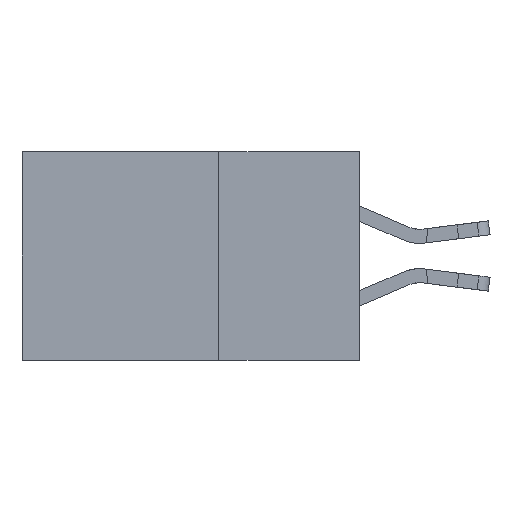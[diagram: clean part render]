
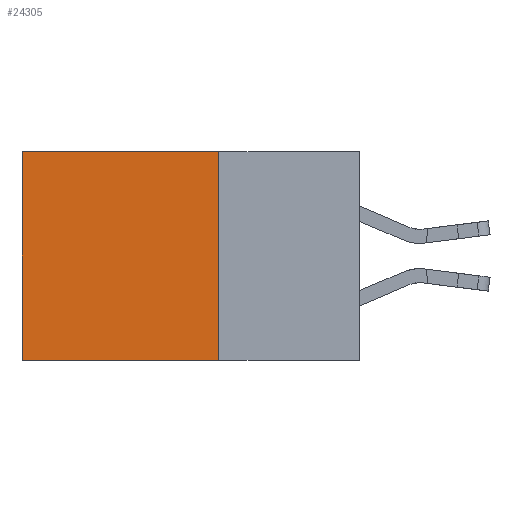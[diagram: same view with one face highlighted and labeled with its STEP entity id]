
A CAD part, left-side view. The second image highlights one B-rep face of the part: STEP entity #24305.
In plain terms, the highlighted planar face has unit normal (-1, 0, 0).
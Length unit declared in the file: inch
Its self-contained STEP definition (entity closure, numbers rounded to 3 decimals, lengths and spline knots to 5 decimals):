
#8 = DIRECTION ( 'NONE',  ( 0., 0., -1. ) ) ;
#394 = EDGE_CURVE ( 'NONE', #16042, #1159, #5912, .T. ) ;
#1159 = VERTEX_POINT ( 'NONE', #7861 ) ;
#1771 = AXIS2_PLACEMENT_3D ( 'NONE', #2518, #14884, #28732 ) ;
#2518 = CARTESIAN_POINT ( 'NONE',  ( 0.2875, 0.25, 0. ) ) ;
#3125 = VECTOR ( 'NONE', #8450, 39.37008 ) ;
#4966 = ORIENTED_EDGE ( 'NONE', *, *, #394, .F. ) ;
#4973 = EDGE_CURVE ( 'NONE', #1159, #19382, #18060, .T. ) ;
#5912 = LINE ( 'NONE', #15812, #14977 ) ;
#7436 = FACE_OUTER_BOUND ( 'NONE', #29350, .T. ) ;
#7861 = CARTESIAN_POINT ( 'NONE',  ( 0.2875, 0.25, -0.37 ) ) ;
#8338 = CARTESIAN_POINT ( 'NONE',  ( 0.2875, 0.25, 0. ) ) ;
#8450 = DIRECTION ( 'NONE',  ( 0., 1., 0. ) ) ;
#11139 = ORIENTED_EDGE ( 'NONE', *, *, #4973, .F. ) ;
#11527 = VERTEX_POINT ( 'NONE', #19496 ) ;
#13624 = VECTOR ( 'NONE', #8, 39.37008 ) ;
#13975 = ORIENTED_EDGE ( 'NONE', *, *, #24794, .T. ) ;
#14884 = DIRECTION ( 'NONE',  ( 1., 0., 0. ) ) ;
#14977 = VECTOR ( 'NONE', #29983, 39.37008 ) ;
#15812 = CARTESIAN_POINT ( 'NONE',  ( 0.2875, 0.25, 0. ) ) ;
#16042 = VERTEX_POINT ( 'NONE', #26250 ) ;
#16046 = CARTESIAN_POINT ( 'NONE',  ( 0.2875, 0.25, -0.37 ) ) ;
#17190 = LINE ( 'NONE', #8338, #20612 ) ;
#18060 = LINE ( 'NONE', #16046, #3125 ) ;
#19020 = CARTESIAN_POINT ( 'NONE',  ( 0.2875, 0.6, 0. ) ) ;
#19382 = VERTEX_POINT ( 'NONE', #22869 ) ;
#19496 = CARTESIAN_POINT ( 'NONE',  ( 0.2875, 0.6, 0. ) ) ;
#20541 = ORIENTED_EDGE ( 'NONE', *, *, #28928, .T. ) ;
#20612 = VECTOR ( 'NONE', #22085, 39.37008 ) ;
#21348 = PLANE ( 'NONE',  #1771 ) ;
#22085 = DIRECTION ( 'NONE',  ( 0., 1., 0. ) ) ;
#22869 = CARTESIAN_POINT ( 'NONE',  ( 0.2875, 0.6, -0.37 ) ) ;
#24305 = ADVANCED_FACE ( 'NONE', ( #7436 ), #21348, .F. ) ;
#24794 = EDGE_CURVE ( 'NONE', #11527, #19382, #26212, .T. ) ;
#26212 = LINE ( 'NONE', #19020, #13624 ) ;
#26250 = CARTESIAN_POINT ( 'NONE',  ( 0.2875, 0.25, 0. ) ) ;
#28732 = DIRECTION ( 'NONE',  ( 0., 0., -1. ) ) ;
#28928 = EDGE_CURVE ( 'NONE', #16042, #11527, #17190, .T. ) ;
#29350 = EDGE_LOOP ( 'NONE', ( #13975, #11139, #4966, #20541 ) ) ;
#29983 = DIRECTION ( 'NONE',  ( 0., 0., -1. ) ) ;
